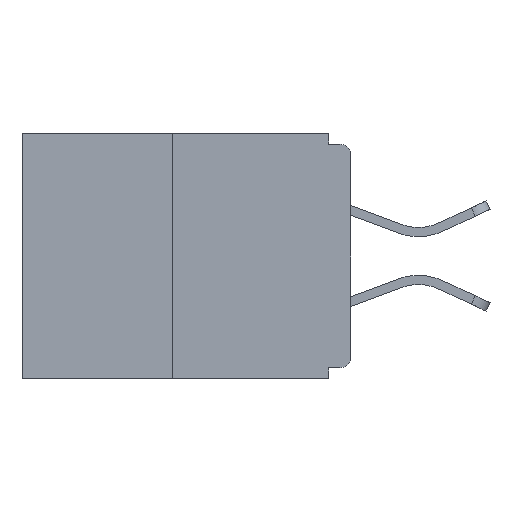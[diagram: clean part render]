
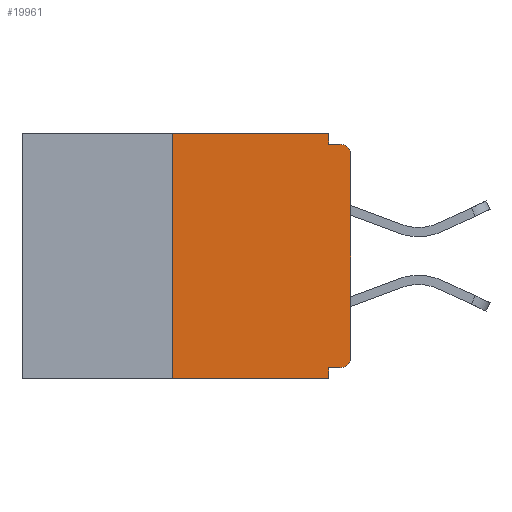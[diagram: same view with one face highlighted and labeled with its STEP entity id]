
A CAD part, left-side view. The second image highlights one B-rep face of the part: STEP entity #19961.
In plain terms, the highlighted planar face has unit normal (-1, 0, 0).
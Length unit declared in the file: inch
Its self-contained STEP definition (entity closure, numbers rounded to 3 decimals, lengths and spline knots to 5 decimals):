
#468 = VERTEX_POINT ( 'NONE', #5515 ) ;
#469 = ORIENTED_EDGE ( 'NONE', *, *, #20257, .F. ) ;
#479 = CIRCLE ( 'NONE', #12738, 0.015 ) ;
#547 = CARTESIAN_POINT ( 'NONE',  ( 0., 0.25, 0. ) ) ;
#1838 = CARTESIAN_POINT ( 'NONE',  ( 0., 0.46, 0. ) ) ;
#1933 = DIRECTION ( 'NONE',  ( 1., 0., 0. ) ) ;
#2547 = CARTESIAN_POINT ( 'NONE',  ( 0., 0.46, -0.343 ) ) ;
#3254 = AXIS2_PLACEMENT_3D ( 'NONE', #1838, #1933, #9402 ) ;
#4035 = VERTEX_POINT ( 'NONE', #11705 ) ;
#5144 = LINE ( 'NONE', #14667, #5514 ) ;
#5514 = VECTOR ( 'NONE', #26429, 39.37008 ) ;
#5515 = CARTESIAN_POINT ( 'NONE',  ( 0., 0.25, -0.343 ) ) ;
#5543 = CARTESIAN_POINT ( 'NONE',  ( 0., 0.031, 0. ) ) ;
#5557 = DIRECTION ( 'NONE',  ( 0., -1., 0. ) ) ;
#5624 = DIRECTION ( 'NONE',  ( 0., 0., -1. ) ) ;
#5703 = EDGE_CURVE ( 'NONE', #20608, #24535, #5144, .T. ) ;
#5892 = EDGE_CURVE ( 'NONE', #468, #21841, #13790, .T. ) ;
#6097 = ORIENTED_EDGE ( 'NONE', *, *, #5892, .F. ) ;
#6145 = VECTOR ( 'NONE', #10325, 39.37008 ) ;
#6658 = DIRECTION ( 'NONE',  ( 0., 0., -1. ) ) ;
#6680 = EDGE_CURVE ( 'NONE', #22344, #16953, #10792, .T. ) ;
#7608 = LINE ( 'NONE', #11666, #14480 ) ;
#7842 = DIRECTION ( 'NONE',  ( 0., 0., -1. ) ) ;
#7978 = VECTOR ( 'NONE', #14276, 39.37008 ) ;
#8702 = VECTOR ( 'NONE', #23120, 39.37008 ) ;
#9369 = EDGE_LOOP ( 'NONE', ( #27317, #6097, #11072, #26746, #23071, #14715, #10881, #17080, #14464, #469 ) ) ;
#9382 = LINE ( 'NONE', #19315, #27799 ) ;
#9402 = DIRECTION ( 'NONE',  ( 0., 0., -1. ) ) ;
#9818 = CARTESIAN_POINT ( 'NONE',  ( 0., 0.015, -0.313 ) ) ;
#10062 = DIRECTION ( 'NONE',  ( 0., 0., -1. ) ) ;
#10325 = DIRECTION ( 'NONE',  ( 0., -1., 0. ) ) ;
#10792 = LINE ( 'NONE', #17593, #6145 ) ;
#10881 = ORIENTED_EDGE ( 'NONE', *, *, #5703, .T. ) ;
#10967 = CARTESIAN_POINT ( 'NONE',  ( 0., 0.015, -0.03 ) ) ;
#11072 = ORIENTED_EDGE ( 'NONE', *, *, #27460, .T. ) ;
#11666 = CARTESIAN_POINT ( 'NONE',  ( 0., 0., -0.328 ) ) ;
#11705 = CARTESIAN_POINT ( 'NONE',  ( 0., 0.031, -0.343 ) ) ;
#12365 = PLANE ( 'NONE',  #3254 ) ;
#12664 = LINE ( 'NONE', #2547, #8702 ) ;
#12738 = AXIS2_PLACEMENT_3D ( 'NONE', #9818, #28501, #5624 ) ;
#13089 = VERTEX_POINT ( 'NONE', #18815 ) ;
#13093 = EDGE_CURVE ( 'NONE', #28687, #4035, #21098, .T. ) ;
#13590 = VERTEX_POINT ( 'NONE', #5543 ) ;
#13790 = LINE ( 'NONE', #22291, #7978 ) ;
#14276 = DIRECTION ( 'NONE',  ( 0., 0., 1. ) ) ;
#14464 = ORIENTED_EDGE ( 'NONE', *, *, #6680, .F. ) ;
#14480 = VECTOR ( 'NONE', #23858, 39.37008 ) ;
#14605 = CARTESIAN_POINT ( 'NONE',  ( 0., 0.031, -0.343 ) ) ;
#14667 = CARTESIAN_POINT ( 'NONE',  ( 0., 0., 0. ) ) ;
#14715 = ORIENTED_EDGE ( 'NONE', *, *, #16800, .T. ) ;
#16433 = VECTOR ( 'NONE', #7842, 39.37008 ) ;
#16800 = EDGE_CURVE ( 'NONE', #13089, #20608, #479, .T. ) ;
#16953 = VERTEX_POINT ( 'NONE', #18242 ) ;
#17080 = ORIENTED_EDGE ( 'NONE', *, *, #22256, .T. ) ;
#17096 = CARTESIAN_POINT ( 'NONE',  ( 0., 0.031, -0.328 ) ) ;
#17329 = CARTESIAN_POINT ( 'NONE',  ( 0., 0.031, -0.015 ) ) ;
#17593 = CARTESIAN_POINT ( 'NONE',  ( 0., 0., -0.015 ) ) ;
#17686 = CARTESIAN_POINT ( 'NONE',  ( 0., 0., -0.03 ) ) ;
#18242 = CARTESIAN_POINT ( 'NONE',  ( 0., 0.015, -0.015 ) ) ;
#18815 = CARTESIAN_POINT ( 'NONE',  ( 0., 0.015, -0.328 ) ) ;
#19038 = CARTESIAN_POINT ( 'NONE',  ( 0., 0.031, 0. ) ) ;
#19315 = CARTESIAN_POINT ( 'NONE',  ( 0., 0.46, 0. ) ) ;
#19961 = ADVANCED_FACE ( 'NONE', ( #20743 ), #12365, .F. ) ;
#19983 = VECTOR ( 'NONE', #10062, 39.37008 ) ;
#20097 = CIRCLE ( 'NONE', #24983, 0.015 ) ;
#20257 = EDGE_CURVE ( 'NONE', #13590, #22344, #22514, .T. ) ;
#20608 = VERTEX_POINT ( 'NONE', #29620 ) ;
#20743 = FACE_OUTER_BOUND ( 'NONE', #9369, .T. ) ;
#21098 = LINE ( 'NONE', #14605, #16433 ) ;
#21841 = VERTEX_POINT ( 'NONE', #547 ) ;
#22256 = EDGE_CURVE ( 'NONE', #24535, #16953, #20097, .T. ) ;
#22291 = CARTESIAN_POINT ( 'NONE',  ( 0., 0.25, 0. ) ) ;
#22344 = VERTEX_POINT ( 'NONE', #17329 ) ;
#22514 = LINE ( 'NONE', #19038, #19983 ) ;
#23071 = ORIENTED_EDGE ( 'NONE', *, *, #26917, .F. ) ;
#23120 = DIRECTION ( 'NONE',  ( 0., -1., 0. ) ) ;
#23858 = DIRECTION ( 'NONE',  ( 0., 1., 0. ) ) ;
#24535 = VERTEX_POINT ( 'NONE', #17686 ) ;
#24983 = AXIS2_PLACEMENT_3D ( 'NONE', #10967, #27115, #6658 ) ;
#26429 = DIRECTION ( 'NONE',  ( 0., 0., 1. ) ) ;
#26746 = ORIENTED_EDGE ( 'NONE', *, *, #13093, .F. ) ;
#26917 = EDGE_CURVE ( 'NONE', #13089, #28687, #7608, .T. ) ;
#26999 = EDGE_CURVE ( 'NONE', #21841, #13590, #9382, .T. ) ;
#27115 = DIRECTION ( 'NONE',  ( -1., 0., 0. ) ) ;
#27317 = ORIENTED_EDGE ( 'NONE', *, *, #26999, .F. ) ;
#27460 = EDGE_CURVE ( 'NONE', #468, #4035, #12664, .T. ) ;
#27799 = VECTOR ( 'NONE', #5557, 39.37008 ) ;
#28501 = DIRECTION ( 'NONE',  ( -1., 0., 0. ) ) ;
#28687 = VERTEX_POINT ( 'NONE', #17096 ) ;
#29620 = CARTESIAN_POINT ( 'NONE',  ( 0., 0., -0.313 ) ) ;
